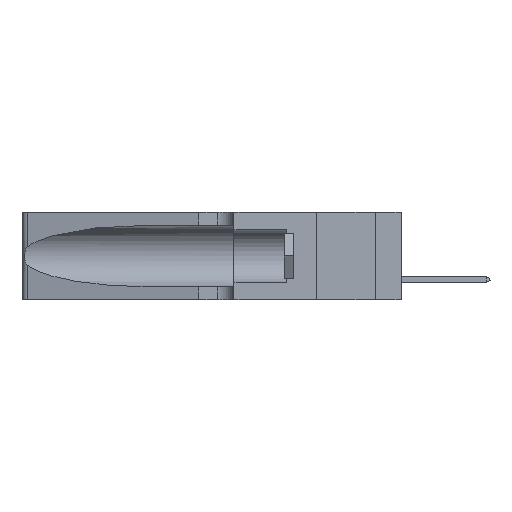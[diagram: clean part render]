
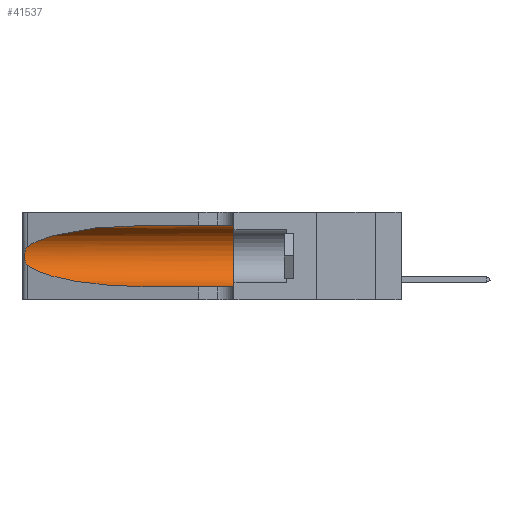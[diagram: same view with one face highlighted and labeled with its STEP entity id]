
A CAD part, left-side view. The second image highlights one B-rep face of the part: STEP entity #41537.
In plain terms, the highlighted cylindrical face has radius 3.308 mm (diameter 6.617 mm), a partial arc.
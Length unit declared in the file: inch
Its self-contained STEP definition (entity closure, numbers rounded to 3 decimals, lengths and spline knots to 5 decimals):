
#93 = EDGE_CURVE ( 'NONE', #41055, #36307, #44373, .T. ) ;
#184 = CARTESIAN_POINT ( 'NONE',  ( 0.26075, 1.23896, 0.19203 ) ) ;
#398 = ORIENTED_EDGE ( 'NONE', *, *, #34448, .T. ) ;
#529 = CARTESIAN_POINT ( 'NONE',  ( 0.25487, 1.22718, 0.14631 ) ) ;
#796 = DIRECTION ( 'NONE',  ( 0., 0., 1. ) ) ;
#948 = ORIENTED_EDGE ( 'NONE', *, *, #25149, .T. ) ;
#2236 = CARTESIAN_POINT ( 'NONE',  ( 0.2373, 1.15595, 0.28018 ) ) ;
#2461 = CARTESIAN_POINT ( 'NONE',  ( 0.25487, 1.22718, 0.22369 ) ) ;
#3598 = AXIS2_PLACEMENT_3D ( 'NONE', #23155, #20940, #796 ) ;
#4297 = CARTESIAN_POINT ( 'NONE',  ( 0.26075, 1.23896, 0.178 ) ) ;
#6184 = CYLINDRICAL_SURFACE ( 'NONE', #12446, 0.13025 ) ;
#6469 = VERTEX_POINT ( 'NONE', #2461 ) ;
#7777 = CARTESIAN_POINT ( 'NONE',  ( 0.25787, 1.23484, 0.2124 ) ) ;
#8282 = CARTESIAN_POINT ( 'NONE',  ( 0.25856, 1.23593, 0.16098 ) ) ;
#8808 = VERTEX_POINT ( 'NONE', #38820 ) ;
#9637 = CARTESIAN_POINT ( 'NONE',  ( 0.1305, 0.35, 0.05475 ) ) ;
#9670 = DIRECTION ( 'NONE',  ( 0., -1., 0. ) ) ;
#12278 = CARTESIAN_POINT ( 'NONE',  ( 0.25555, 1.22994, 0.2215 ) ) ;
#12314 = CARTESIAN_POINT ( 'NONE',  ( 0.25487, 1.22718, 0.14631 ) ) ;
#12446 = AXIS2_PLACEMENT_3D ( 'NONE', #35116, #15727, #23386 ) ;
#15727 = DIRECTION ( 'NONE',  ( 0., -1., 0. ) ) ;
#15971 = VERTEX_POINT ( 'NONE', #9637 ) ;
#16331 = EDGE_LOOP ( 'NONE', ( #36984, #398, #28237, #948, #40988, #21029 ) ) ;
#17612 = EDGE_CURVE ( 'NONE', #41055, #6469, #42492, .T. ) ;
#20287 = CARTESIAN_POINT ( 'NONE',  ( 0.25555, 1.22993, 0.14849 ) ) ;
#20940 = DIRECTION ( 'NONE',  ( 0., 1., 0. ) ) ;
#21025 = EDGE_CURVE ( 'NONE', #36307, #15971, #36353, .T. ) ;
#21029 = ORIENTED_EDGE ( 'NONE', *, *, #93, .F. ) ;
#21456 = LINE ( 'NONE', #27076, #26441 ) ;
#22067 = CARTESIAN_POINT ( 'NONE',  ( 0.2373, 1.15595, 0.08982 ) ) ;
#22898 = CARTESIAN_POINT ( 'NONE',  ( 0.1305, 0.72297, 0.31525 ) ) ;
#23155 = CARTESIAN_POINT ( 'NONE',  ( 0.1305, 0.35, 0.185 ) ) ;
#23386 = DIRECTION ( 'NONE',  ( 0., 0., -1. ) ) ;
#24140 = CARTESIAN_POINT ( 'NONE',  ( 0.26018, 1.23835, 0.19895 ) ) ;
#25036 = EDGE_CURVE ( 'NONE', #37189, #8808, #39339, .T. ) ;
#25149 = EDGE_CURVE ( 'NONE', #8808, #15971, #21456, .T. ) ;
#25620 = CARTESIAN_POINT ( 'NONE',  ( 0.18966, 0.96281, 0.31525 ) ) ;
#25788 = CARTESIAN_POINT ( 'NONE',  ( 0.1305, 0.72297, 0.31525 ) ) ;
#25865 = CARTESIAN_POINT ( 'NONE',  ( 0.1305, 0.72297, 0.05475 ) ) ;
#26441 = VECTOR ( 'NONE', #42961, 39.37008 ) ;
#27076 = CARTESIAN_POINT ( 'NONE',  ( 0.1305, 1.61858, 0.05475 ) ) ;
#27331 = FACE_OUTER_BOUND ( 'NONE', #16331, .T. ) ;
#27908 = B_SPLINE_CURVE_WITH_KNOTS ( 'NONE', 3,
 ( #47889, #12278, #35695, #7777, #43801, #24140, #184, #4297, #32041, #8282, #36033, #40023, #20287, #529 ),
 .UNSPECIFIED., .F., .F.,
 ( 4, 2, 2, 2, 2, 2, 4 ),
 ( 0., 0.00027, 0.00053, 0.00107, 0.0016, 0.00187, 0.00214 ),
 .UNSPECIFIED. ) ;
#28237 = ORIENTED_EDGE ( 'NONE', *, *, #25036, .T. ) ;
#29589 = CARTESIAN_POINT ( 'NONE',  ( 0.25487, 1.22718, 0.22369 ) ) ;
#32041 = CARTESIAN_POINT ( 'NONE',  ( 0.26017, 1.23833, 0.17102 ) ) ;
#33250 = CARTESIAN_POINT ( 'NONE',  ( 0.1305, 1.61858, 0.31525 ) ) ;
#34145 = CARTESIAN_POINT ( 'NONE',  ( 0.18966, 0.96281, 0.05475 ) ) ;
#34448 = EDGE_CURVE ( 'NONE', #6469, #37189, #27908, .T. ) ;
#35116 = CARTESIAN_POINT ( 'NONE',  ( 0.1305, 1.61858, 0.185 ) ) ;
#35695 = CARTESIAN_POINT ( 'NONE',  ( 0.25639, 1.23184, 0.21858 ) ) ;
#36033 = CARTESIAN_POINT ( 'NONE',  ( 0.25789, 1.23486, 0.15765 ) ) ;
#36307 = VERTEX_POINT ( 'NONE', #50150 ) ;
#36353 = CIRCLE ( 'NONE', #3598, 0.13025 ) ;
#36984 = ORIENTED_EDGE ( 'NONE', *, *, #17612, .T. ) ;
#37189 = VERTEX_POINT ( 'NONE', #12314 ) ;
#37445 = CARTESIAN_POINT ( 'NONE',  ( 0.25487, 1.22718, 0.14631 ) ) ;
#38820 = CARTESIAN_POINT ( 'NONE',  ( 0.1305, 0.72297, 0.05475 ) ) ;
#39339 =( BOUNDED_CURVE ( )  B_SPLINE_CURVE ( 3, ( #37445, #22067, #34145, #25865 ),
 .UNSPECIFIED., .F., .F. ) 
 B_SPLINE_CURVE_WITH_KNOTS ( ( 4, 4 ),
 ( 3.44316, 4.71239 ),
 .UNSPECIFIED. ) 
 CURVE ( )  GEOMETRIC_REPRESENTATION_ITEM ( )  RATIONAL_B_SPLINE_CURVE ( ( 1., 0.87, 0.87, 1. ) ) 
 REPRESENTATION_ITEM ( '' )  );
#40023 = CARTESIAN_POINT ( 'NONE',  ( 0.25639, 1.23186, 0.15144 ) ) ;
#40988 = ORIENTED_EDGE ( 'NONE', *, *, #21025, .F. ) ;
#41055 = VERTEX_POINT ( 'NONE', #22898 ) ;
#41537 = ADVANCED_FACE ( 'NONE', ( #27331 ), #6184, .F. ) ;
#42492 =( BOUNDED_CURVE ( )  B_SPLINE_CURVE ( 3, ( #25788, #25620, #2236, #29589 ),
 .UNSPECIFIED., .F., .F. ) 
 B_SPLINE_CURVE_WITH_KNOTS ( ( 4, 4 ),
 ( 1.5708, 2.84003 ),
 .UNSPECIFIED. ) 
 CURVE ( )  GEOMETRIC_REPRESENTATION_ITEM ( )  RATIONAL_B_SPLINE_CURVE ( ( 1., 0.87, 0.87, 1. ) ) 
 REPRESENTATION_ITEM ( '' )  );
#42961 = DIRECTION ( 'NONE',  ( 0., -1., 0. ) ) ;
#43801 = CARTESIAN_POINT ( 'NONE',  ( 0.25854, 1.2359, 0.20912 ) ) ;
#44373 = LINE ( 'NONE', #33250, #51135 ) ;
#47889 = CARTESIAN_POINT ( 'NONE',  ( 0.25487, 1.22718, 0.22369 ) ) ;
#50150 = CARTESIAN_POINT ( 'NONE',  ( 0.1305, 0.35, 0.31525 ) ) ;
#51135 = VECTOR ( 'NONE', #9670, 39.37008 ) ;
